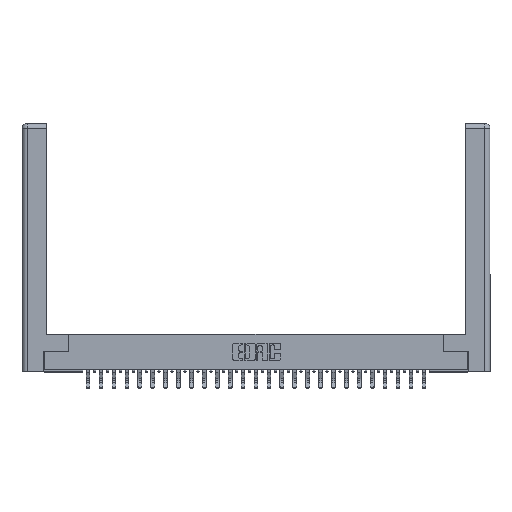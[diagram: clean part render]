
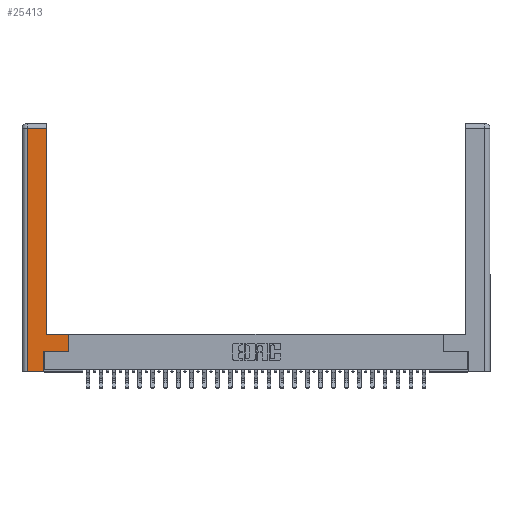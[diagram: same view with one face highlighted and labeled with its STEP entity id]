
A CAD part, top view. The second image highlights one B-rep face of the part: STEP entity #25413.
In plain terms, the highlighted planar face has unit normal (0, 0, 1).
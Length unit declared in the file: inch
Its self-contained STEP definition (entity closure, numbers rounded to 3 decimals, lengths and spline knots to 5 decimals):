
#90 = LINE ( 'NONE', #17015, #14400 ) ;
#138 = EDGE_CURVE ( 'NONE', #26442, #22604, #13778, .T. ) ;
#730 = DIRECTION ( 'NONE',  ( 0., 1., 0. ) ) ;
#1203 = LINE ( 'NONE', #31979, #2832 ) ;
#1525 = VECTOR ( 'NONE', #23796, 39.37008 ) ;
#2377 = VERTEX_POINT ( 'NONE', #11803 ) ;
#2832 = VECTOR ( 'NONE', #31653, 39.37008 ) ;
#2875 = LINE ( 'NONE', #12110, #19253 ) ;
#3975 = DIRECTION ( 'NONE',  ( -1., 0., 0. ) ) ;
#4325 = DIRECTION ( 'NONE',  ( -1., 0., 0. ) ) ;
#4628 = EDGE_LOOP ( 'NONE', ( #24839, #31294, #13505, #32443, #21685, #14200, #29291, #30015 ) ) ;
#5823 = CARTESIAN_POINT ( 'NONE',  ( 0.565, 0.245, 0. ) ) ;
#7137 = CARTESIAN_POINT ( 'NONE',  ( 0.265, 0., 0. ) ) ;
#7408 = CARTESIAN_POINT ( 'NONE',  ( 0.0615, 2.94, 0. ) ) ;
#8606 = EDGE_CURVE ( 'NONE', #33722, #11561, #1203, .T. ) ;
#9099 = CARTESIAN_POINT ( 'NONE',  ( 0.295, 0.45, 0. ) ) ;
#9513 = PLANE ( 'NONE',  #19844 ) ;
#9566 = EDGE_CURVE ( 'NONE', #23812, #26442, #12963, .T. ) ;
#9700 = FACE_OUTER_BOUND ( 'NONE', #4628, .T. ) ;
#9976 = DIRECTION ( 'NONE',  ( 0., 1., 0. ) ) ;
#10512 = CARTESIAN_POINT ( 'NONE',  ( 0.265, 0., 0. ) ) ;
#10636 = VECTOR ( 'NONE', #9976, 39.37008 ) ;
#11113 = EDGE_CURVE ( 'NONE', #11561, #23812, #19375, .T. ) ;
#11561 = VERTEX_POINT ( 'NONE', #28459 ) ;
#11803 = CARTESIAN_POINT ( 'NONE',  ( 0.0615, 0., 0. ) ) ;
#12110 = CARTESIAN_POINT ( 'NONE',  ( 0.565, 0.245, 0. ) ) ;
#12560 = VERTEX_POINT ( 'NONE', #7137 ) ;
#12582 = EDGE_CURVE ( 'NONE', #12560, #18796, #31166, .T. ) ;
#12963 = LINE ( 'NONE', #32085, #19553 ) ;
#13505 = ORIENTED_EDGE ( 'NONE', *, *, #32407, .T. ) ;
#13763 = LINE ( 'NONE', #10512, #1525 ) ;
#13778 = LINE ( 'NONE', #7408, #31861 ) ;
#13802 = CARTESIAN_POINT ( 'NONE',  ( 0.295, 2.94, 0. ) ) ;
#14034 = VECTOR ( 'NONE', #3975, 39.37008 ) ;
#14131 = DIRECTION ( 'NONE',  ( 0., -1., 0. ) ) ;
#14200 = ORIENTED_EDGE ( 'NONE', *, *, #22569, .T. ) ;
#14400 = VECTOR ( 'NONE', #14131, 39.37008 ) ;
#15481 = DIRECTION ( 'NONE',  ( -1., 0., 0. ) ) ;
#17015 = CARTESIAN_POINT ( 'NONE',  ( 0.0615, 0., 0. ) ) ;
#17157 = CARTESIAN_POINT ( 'NONE',  ( 0.295, 0.45, 0. ) ) ;
#17418 = DIRECTION ( 'NONE',  ( 0., 0., -1. ) ) ;
#18796 = VERTEX_POINT ( 'NONE', #21203 ) ;
#19253 = VECTOR ( 'NONE', #33241, 39.37008 ) ;
#19375 = LINE ( 'NONE', #9099, #14034 ) ;
#19553 = VECTOR ( 'NONE', #730, 39.37008 ) ;
#19844 = AXIS2_PLACEMENT_3D ( 'NONE', #27876, #17418, #15481 ) ;
#21203 = CARTESIAN_POINT ( 'NONE',  ( 0.265, 0.245, 0. ) ) ;
#21685 = ORIENTED_EDGE ( 'NONE', *, *, #12582, .T. ) ;
#22569 = EDGE_CURVE ( 'NONE', #18796, #33722, #2875, .T. ) ;
#22604 = VERTEX_POINT ( 'NONE', #25575 ) ;
#23796 = DIRECTION ( 'NONE',  ( 1., 0., 0. ) ) ;
#23812 = VERTEX_POINT ( 'NONE', #17157 ) ;
#24839 = ORIENTED_EDGE ( 'NONE', *, *, #9566, .T. ) ;
#25413 = ADVANCED_FACE ( 'NONE', ( #9700 ), #9513, .F. ) ;
#25575 = CARTESIAN_POINT ( 'NONE',  ( 0.0615, 2.94, 0. ) ) ;
#25914 = EDGE_CURVE ( 'NONE', #2377, #12560, #13763, .T. ) ;
#26442 = VERTEX_POINT ( 'NONE', #13802 ) ;
#27876 = CARTESIAN_POINT ( 'NONE',  ( 0., 0., 0. ) ) ;
#28459 = CARTESIAN_POINT ( 'NONE',  ( 0.565, 0.45, 0. ) ) ;
#29291 = ORIENTED_EDGE ( 'NONE', *, *, #8606, .T. ) ;
#30015 = ORIENTED_EDGE ( 'NONE', *, *, #11113, .T. ) ;
#30725 = CARTESIAN_POINT ( 'NONE',  ( 0.265, 0.245, 0. ) ) ;
#31166 = LINE ( 'NONE', #30725, #10636 ) ;
#31294 = ORIENTED_EDGE ( 'NONE', *, *, #138, .T. ) ;
#31653 = DIRECTION ( 'NONE',  ( 0., 1., 0. ) ) ;
#31861 = VECTOR ( 'NONE', #4325, 39.37008 ) ;
#31979 = CARTESIAN_POINT ( 'NONE',  ( 0.565, 0.45, 0. ) ) ;
#32085 = CARTESIAN_POINT ( 'NONE',  ( 0.295, 3., 0. ) ) ;
#32407 = EDGE_CURVE ( 'NONE', #22604, #2377, #90, .T. ) ;
#32443 = ORIENTED_EDGE ( 'NONE', *, *, #25914, .T. ) ;
#33241 = DIRECTION ( 'NONE',  ( 1., 0., 0. ) ) ;
#33722 = VERTEX_POINT ( 'NONE', #5823 ) ;
